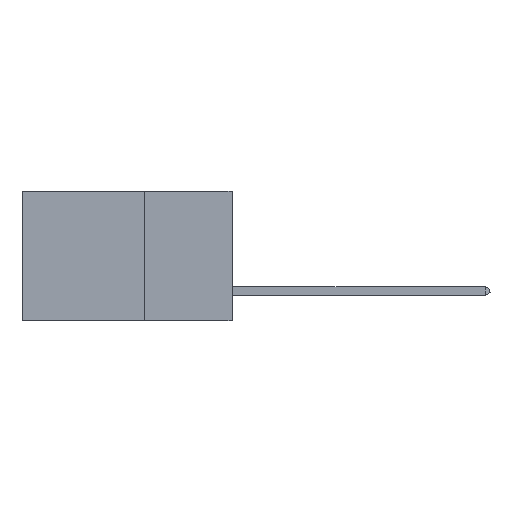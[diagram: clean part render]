
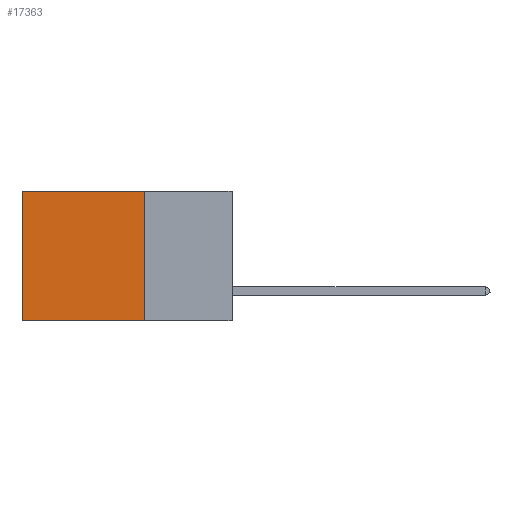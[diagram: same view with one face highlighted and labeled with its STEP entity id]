
A CAD part, left-side view. The second image highlights one B-rep face of the part: STEP entity #17363.
In plain terms, the highlighted planar face has unit normal (-1, 0, 0).
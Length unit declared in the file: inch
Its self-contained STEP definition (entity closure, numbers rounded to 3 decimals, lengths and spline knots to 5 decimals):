
#450 = CARTESIAN_POINT ( 'NONE',  ( 0.2875, 0.25, 0. ) ) ;
#710 = ORIENTED_EDGE ( 'NONE', *, *, #12750, .F. ) ;
#852 = EDGE_LOOP ( 'NONE', ( #15484, #710, #9888, #12518 ) ) ;
#865 = DIRECTION ( 'NONE',  ( 0., 1., 0. ) ) ;
#994 = LINE ( 'NONE', #12683, #8691 ) ;
#1463 = EDGE_CURVE ( 'NONE', #5108, #13291, #14653, .T. ) ;
#1484 = VECTOR ( 'NONE', #5880, 39.37008 ) ;
#2903 = PLANE ( 'NONE',  #16364 ) ;
#3933 = LINE ( 'NONE', #11709, #6265 ) ;
#5108 = VERTEX_POINT ( 'NONE', #15474 ) ;
#5793 = CARTESIAN_POINT ( 'NONE',  ( 0.2875, 0.6, 0. ) ) ;
#5880 = DIRECTION ( 'NONE',  ( 0., 1., 0. ) ) ;
#6081 = EDGE_CURVE ( 'NONE', #5108, #8154, #6397, .T. ) ;
#6265 = VECTOR ( 'NONE', #865, 39.37008 ) ;
#6397 = LINE ( 'NONE', #16756, #1484 ) ;
#7486 = VERTEX_POINT ( 'NONE', #10253 ) ;
#8154 = VERTEX_POINT ( 'NONE', #5793 ) ;
#8165 = CARTESIAN_POINT ( 'NONE',  ( 0.2875, 0.25, 0. ) ) ;
#8608 = EDGE_CURVE ( 'NONE', #8154, #7486, #994, .T. ) ;
#8691 = VECTOR ( 'NONE', #16697, 39.37008 ) ;
#9888 = ORIENTED_EDGE ( 'NONE', *, *, #1463, .F. ) ;
#10253 = CARTESIAN_POINT ( 'NONE',  ( 0.2875, 0.6, -0.37 ) ) ;
#10611 = CARTESIAN_POINT ( 'NONE',  ( 0.2875, 0.25, -0.37 ) ) ;
#10995 = VECTOR ( 'NONE', #12809, 39.37008 ) ;
#11709 = CARTESIAN_POINT ( 'NONE',  ( 0.2875, 0.25, -0.37 ) ) ;
#12518 = ORIENTED_EDGE ( 'NONE', *, *, #6081, .T. ) ;
#12683 = CARTESIAN_POINT ( 'NONE',  ( 0.2875, 0.6, 0. ) ) ;
#12750 = EDGE_CURVE ( 'NONE', #13291, #7486, #3933, .T. ) ;
#12809 = DIRECTION ( 'NONE',  ( 0., 0., -1. ) ) ;
#13291 = VERTEX_POINT ( 'NONE', #10611 ) ;
#13843 = DIRECTION ( 'NONE',  ( 1., 0., 0. ) ) ;
#14653 = LINE ( 'NONE', #450, #10995 ) ;
#14659 = FACE_OUTER_BOUND ( 'NONE', #852, .T. ) ;
#15474 = CARTESIAN_POINT ( 'NONE',  ( 0.2875, 0.25, 0. ) ) ;
#15484 = ORIENTED_EDGE ( 'NONE', *, *, #8608, .T. ) ;
#16364 = AXIS2_PLACEMENT_3D ( 'NONE', #8165, #13843, #16445 ) ;
#16445 = DIRECTION ( 'NONE',  ( 0., 0., -1. ) ) ;
#16697 = DIRECTION ( 'NONE',  ( 0., 0., -1. ) ) ;
#16756 = CARTESIAN_POINT ( 'NONE',  ( 0.2875, 0.25, 0. ) ) ;
#17363 = ADVANCED_FACE ( 'NONE', ( #14659 ), #2903, .F. ) ;
